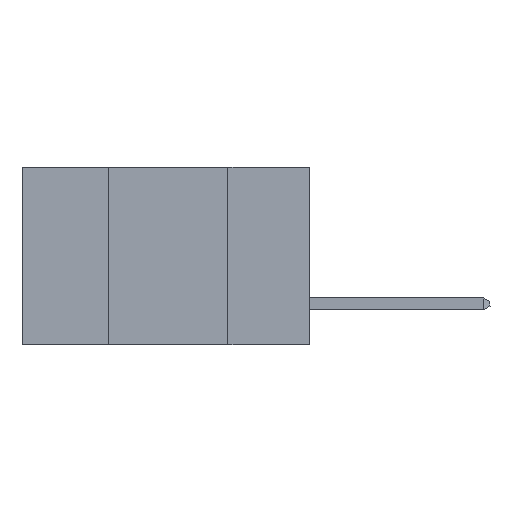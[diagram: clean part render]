
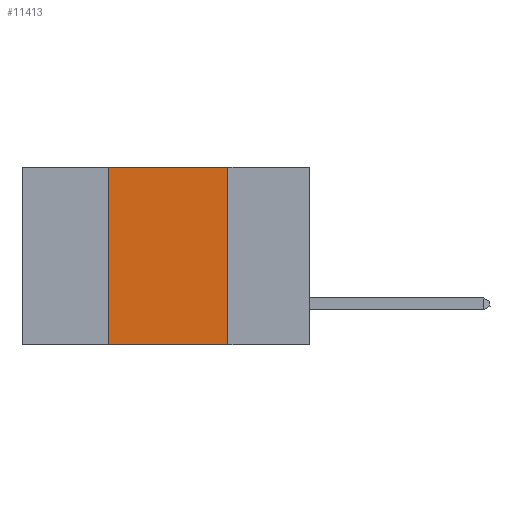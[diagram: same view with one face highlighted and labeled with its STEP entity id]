
A CAD part, left-side view. The second image highlights one B-rep face of the part: STEP entity #11413.
In plain terms, the highlighted planar face has unit normal (-1, 0, 0).
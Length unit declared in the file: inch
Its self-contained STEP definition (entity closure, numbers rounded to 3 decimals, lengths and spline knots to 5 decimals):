
#356 = EDGE_CURVE ( 'NONE', #596, #9218, #866, .T. ) ;
#451 = CARTESIAN_POINT ( 'NONE',  ( 0., 0.17, 0. ) ) ;
#596 = VERTEX_POINT ( 'NONE', #3376 ) ;
#649 = VECTOR ( 'NONE', #9145, 39.37008 ) ;
#673 = VECTOR ( 'NONE', #3615, 39.37008 ) ;
#866 = LINE ( 'NONE', #4828, #12033 ) ;
#1002 = CARTESIAN_POINT ( 'NONE',  ( 0., 0.42, 0. ) ) ;
#1287 = FACE_OUTER_BOUND ( 'NONE', #8484, .T. ) ;
#2739 = LINE ( 'NONE', #1002, #649 ) ;
#2753 = DIRECTION ( 'NONE',  ( 1., 0., 0. ) ) ;
#3376 = CARTESIAN_POINT ( 'NONE',  ( 0., 0.42, -0.37 ) ) ;
#3615 = DIRECTION ( 'NONE',  ( 0., -1., 0. ) ) ;
#3799 = CARTESIAN_POINT ( 'NONE',  ( 0., 0.42, 0. ) ) ;
#3907 = ORIENTED_EDGE ( 'NONE', *, *, #12148, .F. ) ;
#4549 = CARTESIAN_POINT ( 'NONE',  ( 0., 0.6, 0. ) ) ;
#4553 = VERTEX_POINT ( 'NONE', #12163 ) ;
#4828 = CARTESIAN_POINT ( 'NONE',  ( 0., 0.6, -0.37 ) ) ;
#4991 = CARTESIAN_POINT ( 'NONE',  ( 0., 0.6, 0. ) ) ;
#5107 = ORIENTED_EDGE ( 'NONE', *, *, #10986, .F. ) ;
#5851 = PLANE ( 'NONE',  #6238 ) ;
#5918 = DIRECTION ( 'NONE',  ( 0., -1., 0. ) ) ;
#6132 = LINE ( 'NONE', #4549, #673 ) ;
#6238 = AXIS2_PLACEMENT_3D ( 'NONE', #4991, #2753, #10119 ) ;
#7216 = VECTOR ( 'NONE', #11823, 39.37008 ) ;
#7560 = LINE ( 'NONE', #451, #7216 ) ;
#8484 = EDGE_LOOP ( 'NONE', ( #3907, #9585, #5107, #12196 ) ) ;
#9145 = DIRECTION ( 'NONE',  ( 0., 0., 1. ) ) ;
#9218 = VERTEX_POINT ( 'NONE', #12819 ) ;
#9585 = ORIENTED_EDGE ( 'NONE', *, *, #10258, .F. ) ;
#10119 = DIRECTION ( 'NONE',  ( 0., 0., -1. ) ) ;
#10258 = EDGE_CURVE ( 'NONE', #12937, #4553, #6132, .T. ) ;
#10986 = EDGE_CURVE ( 'NONE', #596, #12937, #2739, .T. ) ;
#11413 = ADVANCED_FACE ( 'NONE', ( #1287 ), #5851, .F. ) ;
#11823 = DIRECTION ( 'NONE',  ( 0., 0., -1. ) ) ;
#12033 = VECTOR ( 'NONE', #5918, 39.37008 ) ;
#12148 = EDGE_CURVE ( 'NONE', #4553, #9218, #7560, .T. ) ;
#12163 = CARTESIAN_POINT ( 'NONE',  ( 0., 0.17, 0. ) ) ;
#12196 = ORIENTED_EDGE ( 'NONE', *, *, #356, .T. ) ;
#12819 = CARTESIAN_POINT ( 'NONE',  ( 0., 0.17, -0.37 ) ) ;
#12937 = VERTEX_POINT ( 'NONE', #3799 ) ;
